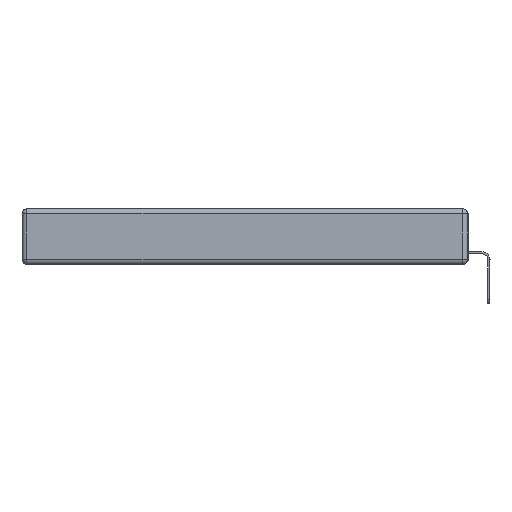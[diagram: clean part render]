
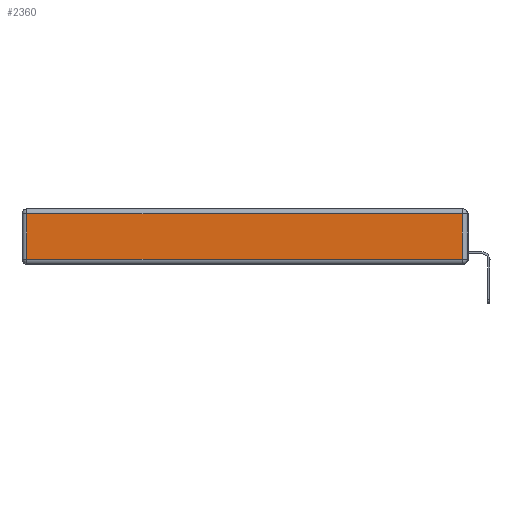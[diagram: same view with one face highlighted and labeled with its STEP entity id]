
A CAD part, left-side view. The second image highlights one B-rep face of the part: STEP entity #2360.
In plain terms, the highlighted planar face has unit normal (-1, 0, 0).
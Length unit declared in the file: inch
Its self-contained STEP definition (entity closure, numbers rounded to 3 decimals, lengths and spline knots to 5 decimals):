
#245 = CARTESIAN_POINT ( 'NONE',  ( 0., 2.72, -0.03 ) ) ;
#499 = ORIENTED_EDGE ( 'NONE', *, *, #14902, .T. ) ;
#1052 = PLANE ( 'NONE',  #18148 ) ;
#1150 = LINE ( 'NONE', #12944, #7697 ) ;
#1633 = CARTESIAN_POINT ( 'NONE',  ( 0., 2.72, -0.313 ) ) ;
#1992 = VECTOR ( 'NONE', #13782, 39.37008 ) ;
#2360 = ADVANCED_FACE ( 'NONE', ( #4370 ), #1052, .T. ) ;
#2525 = ORIENTED_EDGE ( 'NONE', *, *, #16716, .T. ) ;
#3690 = VECTOR ( 'NONE', #11061, 39.37008 ) ;
#4370 = FACE_OUTER_BOUND ( 'NONE', #9494, .T. ) ;
#5051 = DIRECTION ( 'NONE',  ( -1., 0., 0. ) ) ;
#5092 = VERTEX_POINT ( 'NONE', #19637 ) ;
#7200 = DIRECTION ( 'NONE',  ( 0., 0., 1. ) ) ;
#7697 = VECTOR ( 'NONE', #15095, 39.37008 ) ;
#7727 = CARTESIAN_POINT ( 'NONE',  ( 0., 0.03, -0.03 ) ) ;
#7902 = VECTOR ( 'NONE', #21212, 39.37008 ) ;
#9189 = EDGE_CURVE ( 'NONE', #5092, #19928, #17550, .T. ) ;
#9494 = EDGE_LOOP ( 'NONE', ( #2525, #15695, #499, #14173 ) ) ;
#10786 = EDGE_CURVE ( 'NONE', #11083, #11353, #14952, .T. ) ;
#11061 = DIRECTION ( 'NONE',  ( 0., 0., 1. ) ) ;
#11083 = VERTEX_POINT ( 'NONE', #245 ) ;
#11353 = VERTEX_POINT ( 'NONE', #1633 ) ;
#12944 = CARTESIAN_POINT ( 'NONE',  ( 0., 0., -0.313 ) ) ;
#13685 = CARTESIAN_POINT ( 'NONE',  ( 0., 2.72, -0.343 ) ) ;
#13782 = DIRECTION ( 'NONE',  ( 0., 1., 0. ) ) ;
#14173 = ORIENTED_EDGE ( 'NONE', *, *, #10786, .T. ) ;
#14861 = CARTESIAN_POINT ( 'NONE',  ( 0., 0., -0.343 ) ) ;
#14902 = EDGE_CURVE ( 'NONE', #19928, #11083, #22475, .T. ) ;
#14952 = LINE ( 'NONE', #13685, #7902 ) ;
#15095 = DIRECTION ( 'NONE',  ( 0., -1., 0. ) ) ;
#15648 = CARTESIAN_POINT ( 'NONE',  ( 0., 2.75, -0.03 ) ) ;
#15695 = ORIENTED_EDGE ( 'NONE', *, *, #9189, .T. ) ;
#16716 = EDGE_CURVE ( 'NONE', #11353, #5092, #1150, .T. ) ;
#17550 = LINE ( 'NONE', #22820, #3690 ) ;
#18148 = AXIS2_PLACEMENT_3D ( 'NONE', #14861, #5051, #7200 ) ;
#19637 = CARTESIAN_POINT ( 'NONE',  ( 0., 0.03, -0.313 ) ) ;
#19928 = VERTEX_POINT ( 'NONE', #7727 ) ;
#21212 = DIRECTION ( 'NONE',  ( 0., 0., -1. ) ) ;
#22475 = LINE ( 'NONE', #15648, #1992 ) ;
#22820 = CARTESIAN_POINT ( 'NONE',  ( 0., 0.03, -0.343 ) ) ;
